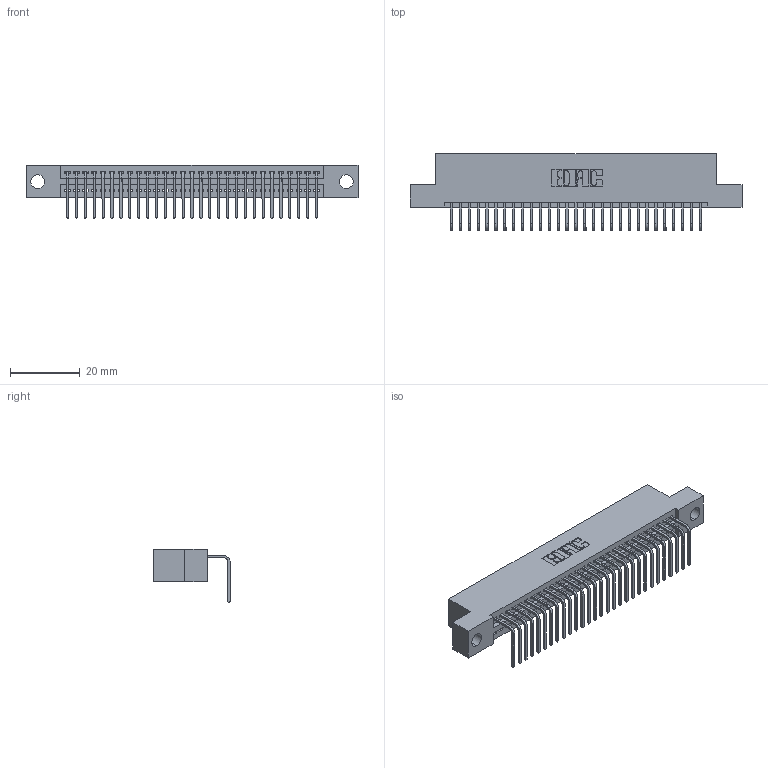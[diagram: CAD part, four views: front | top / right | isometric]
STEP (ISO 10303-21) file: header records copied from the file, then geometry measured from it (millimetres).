
FILE_DESCRIPTION (( 'STEP AP203' ), '1' );
FILE_NAME ('395-029-558-104.STEP', '2018-11-10T21:18:24', ( '' ), ( '' ), 'SwSTEP 2.0', 'SolidWorks 2016', '' );
FILE_SCHEMA (( 'CONFIG_CONTROL_DESIGN' ));
Length unit declared in the file: inch
Products named in the file (3): 345 Part_Flush Mounting Lugs - 0.156 Dia-TH; 395-029-558-104; 345-292-001_558 Tail - 2
Assembly tree (30 placements, depth 2):
  395-029-558-104
    345 Part_Flush Mounting Lugs - 0.156 Dia-TH
    345-292-001_558 Tail - 2  x29
Bounding box: 94.87 x 21.83 x 15.37 mm (x, y, z)
Volume: 8913 mm3; surface area: 12044.4 mm2
Topology: 30 solids, 30 shells, 1866 faces, 5619 edges, 3706 vertices
Faces by surface type: plane 1298, cylinder 568
Entity records: 23663 total; most frequent: CARTESIAN_POINT 4107, ORIENTED_EDGE 4070, DIRECTION 3605, EDGE_CURVE 2035, LINE 1787, VECTOR 1787, VERTEX_POINT 1354, AXIS2_PLACEMENT_3D 909
